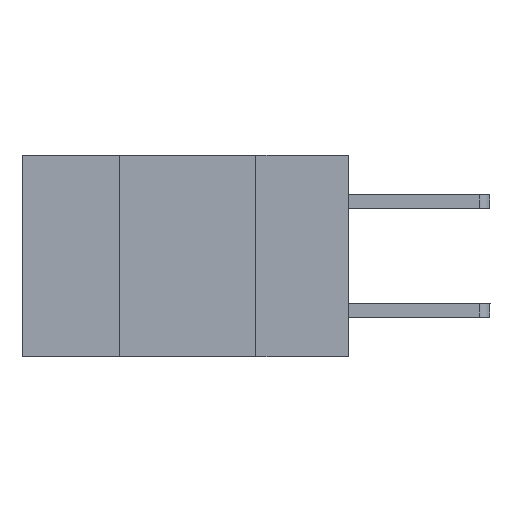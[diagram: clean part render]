
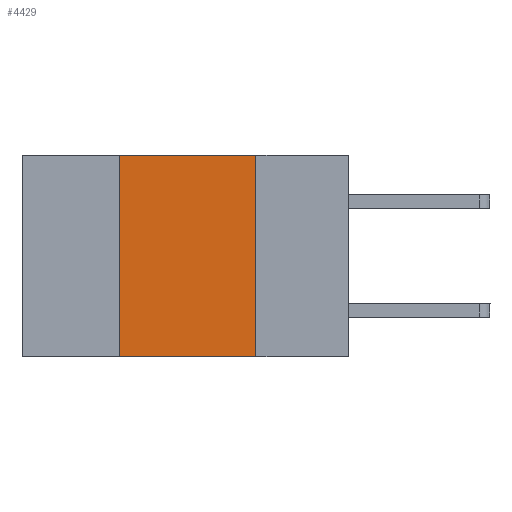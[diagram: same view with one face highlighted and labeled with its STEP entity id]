
A CAD part, left-side view. The second image highlights one B-rep face of the part: STEP entity #4429.
In plain terms, the highlighted planar face has unit normal (-1, 0, 0).
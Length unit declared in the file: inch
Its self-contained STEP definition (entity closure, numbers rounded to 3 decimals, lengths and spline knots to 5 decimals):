
#209 = VECTOR ( 'NONE', #3276, 39.37008 ) ;
#484 = EDGE_CURVE ( 'NONE', #6152, #7317, #4390, .T. ) ;
#490 = EDGE_CURVE ( 'NONE', #3587, #6152, #6061, .T. ) ;
#493 = EDGE_CURVE ( 'NONE', #7620, #3587, #7472, .T. ) ;
#494 = EDGE_CURVE ( 'NONE', #7620, #7317, #8917, .T. ) ;
#857 = CARTESIAN_POINT ( 'NONE',  ( 0., 0.17, -0.37 ) ) ;
#1516 = ORIENTED_EDGE ( 'NONE', *, *, #494, .T. ) ;
#1658 = DIRECTION ( 'NONE',  ( 1., 0., 0. ) ) ;
#2009 = VECTOR ( 'NONE', #2094, 39.37008 ) ;
#2094 = DIRECTION ( 'NONE',  ( 0., -1., 0. ) ) ;
#2829 = CARTESIAN_POINT ( 'NONE',  ( 0., 0.17, 0. ) ) ;
#3213 = FACE_OUTER_BOUND ( 'NONE', #4403, .T. ) ;
#3276 = DIRECTION ( 'NONE',  ( 0., -1., 0. ) ) ;
#3303 = AXIS2_PLACEMENT_3D ( 'NONE', #9051, #1658, #6869 ) ;
#3550 = CARTESIAN_POINT ( 'NONE',  ( 0., 0.42, -0.37 ) ) ;
#3587 = VERTEX_POINT ( 'NONE', #3669 ) ;
#3669 = CARTESIAN_POINT ( 'NONE',  ( 0., 0.42, 0. ) ) ;
#4114 = VECTOR ( 'NONE', #6865, 39.37008 ) ;
#4390 = LINE ( 'NONE', #857, #4114 ) ;
#4403 = EDGE_LOOP ( 'NONE', ( #4547, #8602, #8347, #1516 ) ) ;
#4429 = ADVANCED_FACE ( 'NONE', ( #3213 ), #4886, .F. ) ;
#4547 = ORIENTED_EDGE ( 'NONE', *, *, #484, .F. ) ;
#4886 = PLANE ( 'NONE',  #3303 ) ;
#5663 = CARTESIAN_POINT ( 'NONE',  ( 0., 0.6, 0. ) ) ;
#5674 = CARTESIAN_POINT ( 'NONE',  ( 0., 0.42, -0.37 ) ) ;
#5854 = VECTOR ( 'NONE', #6922, 39.37008 ) ;
#6061 = LINE ( 'NONE', #5663, #209 ) ;
#6152 = VERTEX_POINT ( 'NONE', #2829 ) ;
#6458 = CARTESIAN_POINT ( 'NONE',  ( 0., 0.6, -0.37 ) ) ;
#6483 = CARTESIAN_POINT ( 'NONE',  ( 0., 0.17, -0.37 ) ) ;
#6865 = DIRECTION ( 'NONE',  ( 0., 0., -1. ) ) ;
#6869 = DIRECTION ( 'NONE',  ( 0., 0., -1. ) ) ;
#6922 = DIRECTION ( 'NONE',  ( 0., 0., 1. ) ) ;
#7317 = VERTEX_POINT ( 'NONE', #6483 ) ;
#7472 = LINE ( 'NONE', #3550, #5854 ) ;
#7620 = VERTEX_POINT ( 'NONE', #5674 ) ;
#8347 = ORIENTED_EDGE ( 'NONE', *, *, #493, .F. ) ;
#8602 = ORIENTED_EDGE ( 'NONE', *, *, #490, .F. ) ;
#8917 = LINE ( 'NONE', #6458, #2009 ) ;
#9051 = CARTESIAN_POINT ( 'NONE',  ( 0., 0.6, 0. ) ) ;
